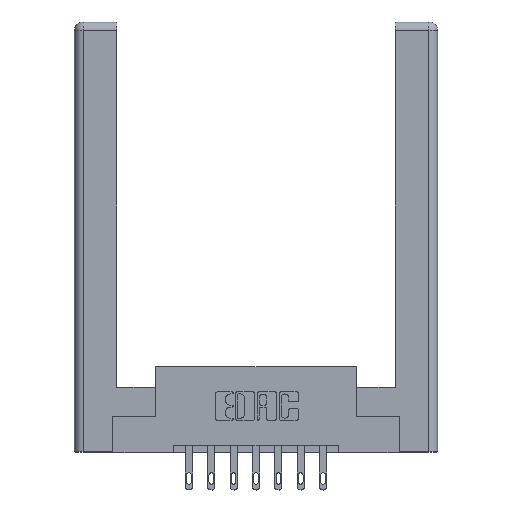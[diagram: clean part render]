
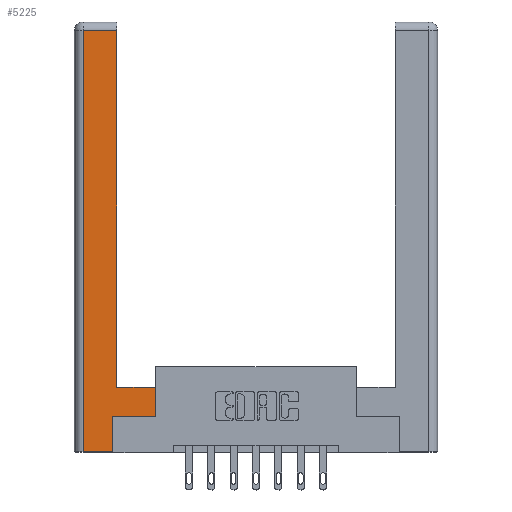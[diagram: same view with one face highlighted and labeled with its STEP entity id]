
A CAD part, top view. The second image highlights one B-rep face of the part: STEP entity #5225.
In plain terms, the highlighted planar face has unit normal (0, 0, 1).
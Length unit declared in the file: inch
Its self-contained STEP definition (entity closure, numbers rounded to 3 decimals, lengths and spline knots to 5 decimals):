
#442 = VECTOR ( 'NONE', #11324, 39.37008 ) ;
#456 = EDGE_CURVE ( 'NONE', #8174, #3191, #5801, .T. ) ;
#634 = DIRECTION ( 'NONE',  ( 0., 0., -1. ) ) ;
#635 = VECTOR ( 'NONE', #11561, 39.37008 ) ;
#841 = FACE_OUTER_BOUND ( 'NONE', #3913, .T. ) ;
#858 = ORIENTED_EDGE ( 'NONE', *, *, #7624, .T. ) ;
#1181 = VERTEX_POINT ( 'NONE', #1319 ) ;
#1319 = CARTESIAN_POINT ( 'NONE',  ( 0.565, 0.245, 0. ) ) ;
#1577 = CARTESIAN_POINT ( 'NONE',  ( 0.265, 0., 0. ) ) ;
#1606 = DIRECTION ( 'NONE',  ( -1., 0., 0. ) ) ;
#1695 = LINE ( 'NONE', #9561, #635 ) ;
#2029 = CARTESIAN_POINT ( 'NONE',  ( 0.0615, 0., 0. ) ) ;
#2357 = EDGE_CURVE ( 'NONE', #3798, #3871, #1695, .T. ) ;
#2601 = PLANE ( 'NONE',  #4730 ) ;
#2654 = CARTESIAN_POINT ( 'NONE',  ( 0.565, 0.45, 0. ) ) ;
#3155 = ORIENTED_EDGE ( 'NONE', *, *, #4267, .T. ) ;
#3191 = VERTEX_POINT ( 'NONE', #9748 ) ;
#3279 = VECTOR ( 'NONE', #11422, 39.37008 ) ;
#3287 = CARTESIAN_POINT ( 'NONE',  ( 0.565, 0.45, 0. ) ) ;
#3571 = CARTESIAN_POINT ( 'NONE',  ( 0.295, 3., 0. ) ) ;
#3769 = EDGE_CURVE ( 'NONE', #3871, #8174, #5706, .T. ) ;
#3798 = VERTEX_POINT ( 'NONE', #2654 ) ;
#3871 = VERTEX_POINT ( 'NONE', #7720 ) ;
#3913 = EDGE_LOOP ( 'NONE', ( #8817, #6423, #12504, #8131, #10567, #3155, #858, #8337 ) ) ;
#4096 = CARTESIAN_POINT ( 'NONE',  ( 0.295, 2.94, 0. ) ) ;
#4267 = EDGE_CURVE ( 'NONE', #10758, #1181, #9475, .T. ) ;
#4427 = DIRECTION ( 'NONE',  ( 1., 0., 0. ) ) ;
#4730 = AXIS2_PLACEMENT_3D ( 'NONE', #9365, #634, #1606 ) ;
#4786 = VECTOR ( 'NONE', #5055, 39.37008 ) ;
#4943 = CARTESIAN_POINT ( 'NONE',  ( 0.0615, 0., 0. ) ) ;
#5055 = DIRECTION ( 'NONE',  ( 1., 0., 0. ) ) ;
#5225 = ADVANCED_FACE ( 'NONE', ( #841 ), #2601, .F. ) ;
#5297 = LINE ( 'NONE', #9913, #11049 ) ;
#5706 = LINE ( 'NONE', #3571, #442 ) ;
#5801 = LINE ( 'NONE', #11223, #3279 ) ;
#5934 = CARTESIAN_POINT ( 'NONE',  ( 0.565, 0.245, 0. ) ) ;
#6264 = CARTESIAN_POINT ( 'NONE',  ( 0.265, 0.245, 0. ) ) ;
#6423 = ORIENTED_EDGE ( 'NONE', *, *, #456, .T. ) ;
#6572 = VECTOR ( 'NONE', #11671, 39.37008 ) ;
#6807 = VECTOR ( 'NONE', #4427, 39.37008 ) ;
#6930 = VERTEX_POINT ( 'NONE', #1577 ) ;
#7342 = LINE ( 'NONE', #4943, #6572 ) ;
#7505 = EDGE_CURVE ( 'NONE', #3191, #10434, #7342, .T. ) ;
#7624 = EDGE_CURVE ( 'NONE', #1181, #3798, #11111, .T. ) ;
#7720 = CARTESIAN_POINT ( 'NONE',  ( 0.295, 0.45, 0. ) ) ;
#8060 = CARTESIAN_POINT ( 'NONE',  ( 0.265, 0., 0. ) ) ;
#8131 = ORIENTED_EDGE ( 'NONE', *, *, #10180, .T. ) ;
#8174 = VERTEX_POINT ( 'NONE', #4096 ) ;
#8195 = LINE ( 'NONE', #8060, #6807 ) ;
#8337 = ORIENTED_EDGE ( 'NONE', *, *, #2357, .T. ) ;
#8817 = ORIENTED_EDGE ( 'NONE', *, *, #3769, .T. ) ;
#9365 = CARTESIAN_POINT ( 'NONE',  ( 0., 0., 0. ) ) ;
#9475 = LINE ( 'NONE', #5934, #4786 ) ;
#9561 = CARTESIAN_POINT ( 'NONE',  ( 0.295, 0.45, 0. ) ) ;
#9748 = CARTESIAN_POINT ( 'NONE',  ( 0.0615, 2.94, 0. ) ) ;
#9913 = CARTESIAN_POINT ( 'NONE',  ( 0.265, 0.245, 0. ) ) ;
#10069 = DIRECTION ( 'NONE',  ( 0., 1., 0. ) ) ;
#10077 = EDGE_CURVE ( 'NONE', #6930, #10758, #5297, .T. ) ;
#10180 = EDGE_CURVE ( 'NONE', #10434, #6930, #8195, .T. ) ;
#10365 = VECTOR ( 'NONE', #10069, 39.37008 ) ;
#10434 = VERTEX_POINT ( 'NONE', #2029 ) ;
#10567 = ORIENTED_EDGE ( 'NONE', *, *, #10077, .T. ) ;
#10758 = VERTEX_POINT ( 'NONE', #6264 ) ;
#10881 = DIRECTION ( 'NONE',  ( 0., 1., 0. ) ) ;
#11049 = VECTOR ( 'NONE', #10881, 39.37008 ) ;
#11111 = LINE ( 'NONE', #3287, #10365 ) ;
#11223 = CARTESIAN_POINT ( 'NONE',  ( 0.0615, 2.94, 0. ) ) ;
#11324 = DIRECTION ( 'NONE',  ( 0., 1., 0. ) ) ;
#11422 = DIRECTION ( 'NONE',  ( -1., 0., 0. ) ) ;
#11561 = DIRECTION ( 'NONE',  ( -1., 0., 0. ) ) ;
#11671 = DIRECTION ( 'NONE',  ( 0., -1., 0. ) ) ;
#12504 = ORIENTED_EDGE ( 'NONE', *, *, #7505, .T. ) ;
